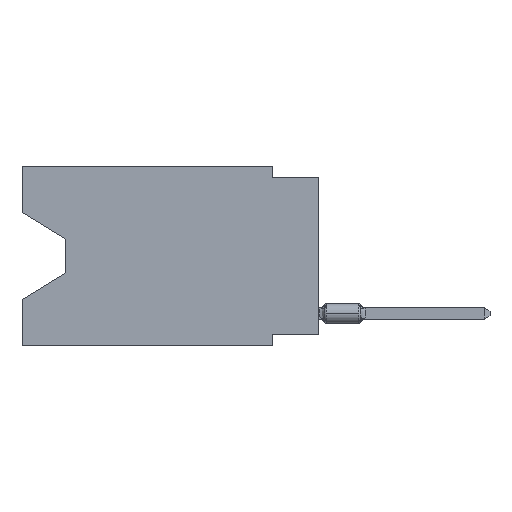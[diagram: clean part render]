
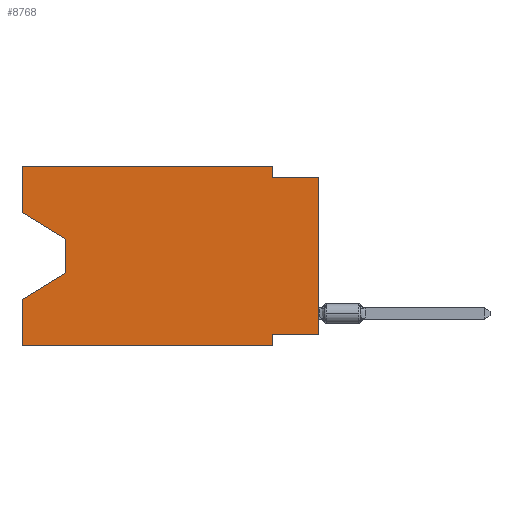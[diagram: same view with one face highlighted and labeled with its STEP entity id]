
A CAD part, left-side view. The second image highlights one B-rep face of the part: STEP entity #8768.
In plain terms, the highlighted planar face has unit normal (-1, 0, 0).
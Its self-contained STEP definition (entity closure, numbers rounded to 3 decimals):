
#216 = VERTEX_POINT ( 'NONE', #17765 ) ;
#1125 = CARTESIAN_POINT ( 'NONE',  ( 0., 0., -9.271 ) ) ;
#1275 = LINE ( 'NONE', #5152, #13679 ) ;
#1315 = VECTOR ( 'NONE', #11865, 1000. ) ;
#1495 = ORIENTED_EDGE ( 'NONE', *, *, #1840, .T. ) ;
#1608 = DIRECTION ( 'NONE',  ( 0., -1., 0. ) ) ;
#1840 = EDGE_CURVE ( 'NONE', #7908, #9397, #9625, .T. ) ;
#1985 = VERTEX_POINT ( 'NONE', #17599 ) ;
#2200 = VERTEX_POINT ( 'NONE', #10750 ) ;
#2422 = LINE ( 'NONE', #6221, #1315 ) ;
#2593 = CARTESIAN_POINT ( 'NONE',  ( 0., 13.97, -5.893 ) ) ;
#2665 = VECTOR ( 'NONE', #6496, 1000. ) ;
#2849 = EDGE_CURVE ( 'NONE', #6398, #18289, #8085, .T. ) ;
#3055 = VERTEX_POINT ( 'NONE', #4558 ) ;
#3320 = ORIENTED_EDGE ( 'NONE', *, *, #4795, .T. ) ;
#3359 = VECTOR ( 'NONE', #12506, 1000. ) ;
#3382 = ORIENTED_EDGE ( 'NONE', *, *, #9108, .F. ) ;
#3465 = CARTESIAN_POINT ( 'NONE',  ( 0., 2.54, 0. ) ) ;
#3468 = CARTESIAN_POINT ( 'NONE',  ( 0., 0., -0.635 ) ) ;
#3696 = VECTOR ( 'NONE', #5291, 1000. ) ;
#3837 = EDGE_LOOP ( 'NONE', ( #6794, #5334, #1495, #3382, #12993, #16751, #5010, #3320, #12485, #5876, #5264, #15847 ) ) ;
#3975 = VECTOR ( 'NONE', #1608, 1000. ) ;
#4051 = VERTEX_POINT ( 'NONE', #5047 ) ;
#4202 = CARTESIAN_POINT ( 'NONE',  ( 0., 16.383, 0. ) ) ;
#4558 = CARTESIAN_POINT ( 'NONE',  ( 0., 0., -0.635 ) ) ;
#4795 = EDGE_CURVE ( 'NONE', #6863, #3055, #7858, .T. ) ;
#4955 = CARTESIAN_POINT ( 'NONE',  ( 0., 13.97, -4.013 ) ) ;
#5010 = ORIENTED_EDGE ( 'NONE', *, *, #12832, .F. ) ;
#5047 = CARTESIAN_POINT ( 'NONE',  ( 0., 2.54, -9.906 ) ) ;
#5059 = DIRECTION ( 'NONE',  ( 1., 0., 0. ) ) ;
#5152 = CARTESIAN_POINT ( 'NONE',  ( 0., 16.383, -9.906 ) ) ;
#5264 = ORIENTED_EDGE ( 'NONE', *, *, #2849, .F. ) ;
#5291 = DIRECTION ( 'NONE',  ( 0., 0., -1. ) ) ;
#5334 = ORIENTED_EDGE ( 'NONE', *, *, #16260, .T. ) ;
#5782 = DIRECTION ( 'NONE',  ( 0., -0.855, -0.519 ) ) ;
#5876 = ORIENTED_EDGE ( 'NONE', *, *, #6886, .F. ) ;
#6113 = CARTESIAN_POINT ( 'NONE',  ( 0., 16.383, -7.36 ) ) ;
#6221 = CARTESIAN_POINT ( 'NONE',  ( 0., 2.54, -9.906 ) ) ;
#6259 = EDGE_CURVE ( 'NONE', #216, #3055, #17273, .T. ) ;
#6398 = VERTEX_POINT ( 'NONE', #16338 ) ;
#6496 = DIRECTION ( 'NONE',  ( 0., 0., 1. ) ) ;
#6783 = CARTESIAN_POINT ( 'NONE',  ( 0., 16.383, 0. ) ) ;
#6794 = ORIENTED_EDGE ( 'NONE', *, *, #14315, .T. ) ;
#6863 = VERTEX_POINT ( 'NONE', #15298 ) ;
#6886 = EDGE_CURVE ( 'NONE', #18289, #216, #7054, .T. ) ;
#7054 = LINE ( 'NONE', #9828, #3696 ) ;
#7429 = VERTEX_POINT ( 'NONE', #4955 ) ;
#7659 = CARTESIAN_POINT ( 'NONE',  ( 0., 16.383, 0. ) ) ;
#7858 = LINE ( 'NONE', #13500, #18079 ) ;
#7908 = VERTEX_POINT ( 'NONE', #12144 ) ;
#8012 = CARTESIAN_POINT ( 'NONE',  ( 0., 16.383, 0. ) ) ;
#8085 = LINE ( 'NONE', #4202, #3975 ) ;
#8768 = ADVANCED_FACE ( 'NONE', ( #17734 ), #14885, .F. ) ;
#8933 = DIRECTION ( 'NONE',  ( 0., -1., 0. ) ) ;
#9108 = EDGE_CURVE ( 'NONE', #1985, #9397, #17978, .T. ) ;
#9397 = VERTEX_POINT ( 'NONE', #6113 ) ;
#9408 = DIRECTION ( 'NONE',  ( 0., -1., 0. ) ) ;
#9625 = LINE ( 'NONE', #2593, #3359 ) ;
#9828 = CARTESIAN_POINT ( 'NONE',  ( 0., 2.54, 0. ) ) ;
#10456 = EDGE_CURVE ( 'NONE', #1985, #4051, #1275, .T. ) ;
#10739 = DIRECTION ( 'NONE',  ( 0., 1., 0. ) ) ;
#10750 = CARTESIAN_POINT ( 'NONE',  ( 0., 16.383, -2.546 ) ) ;
#10891 = EDGE_CURVE ( 'NONE', #2200, #6398, #16623, .T. ) ;
#10926 = DIRECTION ( 'NONE',  ( 0., 0., -1. ) ) ;
#11019 = LINE ( 'NONE', #1125, #14485 ) ;
#11113 = CARTESIAN_POINT ( 'NONE',  ( 0., 13.97, -4.013 ) ) ;
#11865 = DIRECTION ( 'NONE',  ( 0., 0., -1. ) ) ;
#12144 = CARTESIAN_POINT ( 'NONE',  ( 0., 13.97, -5.893 ) ) ;
#12485 = ORIENTED_EDGE ( 'NONE', *, *, #6259, .F. ) ;
#12506 = DIRECTION ( 'NONE',  ( 0., 0.855, -0.519 ) ) ;
#12576 = VECTOR ( 'NONE', #10926, 1000. ) ;
#12832 = EDGE_CURVE ( 'NONE', #6863, #18278, #11019, .T. ) ;
#12993 = ORIENTED_EDGE ( 'NONE', *, *, #10456, .T. ) ;
#13311 = DIRECTION ( 'NONE',  ( 0., 0., -1. ) ) ;
#13500 = CARTESIAN_POINT ( 'NONE',  ( 0., 0., 0. ) ) ;
#13679 = VECTOR ( 'NONE', #9408, 1000. ) ;
#13929 = LINE ( 'NONE', #18280, #17804 ) ;
#14315 = EDGE_CURVE ( 'NONE', #2200, #7429, #13929, .T. ) ;
#14485 = VECTOR ( 'NONE', #10739, 1000. ) ;
#14573 = EDGE_CURVE ( 'NONE', #18278, #4051, #2422, .T. ) ;
#14613 = VECTOR ( 'NONE', #16722, 1000. ) ;
#14630 = VECTOR ( 'NONE', #8933, 1000. ) ;
#14679 = CARTESIAN_POINT ( 'NONE',  ( 0., 2.54, -9.271 ) ) ;
#14885 = PLANE ( 'NONE',  #17151 ) ;
#15298 = CARTESIAN_POINT ( 'NONE',  ( 0., 0., -9.271 ) ) ;
#15847 = ORIENTED_EDGE ( 'NONE', *, *, #10891, .F. ) ;
#16260 = EDGE_CURVE ( 'NONE', #7429, #7908, #18140, .T. ) ;
#16338 = CARTESIAN_POINT ( 'NONE',  ( 0., 16.383, 0. ) ) ;
#16623 = LINE ( 'NONE', #8012, #14613 ) ;
#16722 = DIRECTION ( 'NONE',  ( 0., 0., 1. ) ) ;
#16751 = ORIENTED_EDGE ( 'NONE', *, *, #14573, .F. ) ;
#17151 = AXIS2_PLACEMENT_3D ( 'NONE', #7659, #5059, #13311 ) ;
#17273 = LINE ( 'NONE', #3468, #14630 ) ;
#17568 = DIRECTION ( 'NONE',  ( 0., 0., 1. ) ) ;
#17599 = CARTESIAN_POINT ( 'NONE',  ( 0., 16.383, -9.906 ) ) ;
#17734 = FACE_OUTER_BOUND ( 'NONE', #3837, .T. ) ;
#17765 = CARTESIAN_POINT ( 'NONE',  ( 0., 2.54, -0.635 ) ) ;
#17804 = VECTOR ( 'NONE', #5782, 1000. ) ;
#17978 = LINE ( 'NONE', #6783, #2665 ) ;
#18079 = VECTOR ( 'NONE', #17568, 1000. ) ;
#18140 = LINE ( 'NONE', #11113, #12576 ) ;
#18278 = VERTEX_POINT ( 'NONE', #14679 ) ;
#18280 = CARTESIAN_POINT ( 'NONE',  ( 0., 16.383, -2.546 ) ) ;
#18289 = VERTEX_POINT ( 'NONE', #3465 ) ;
